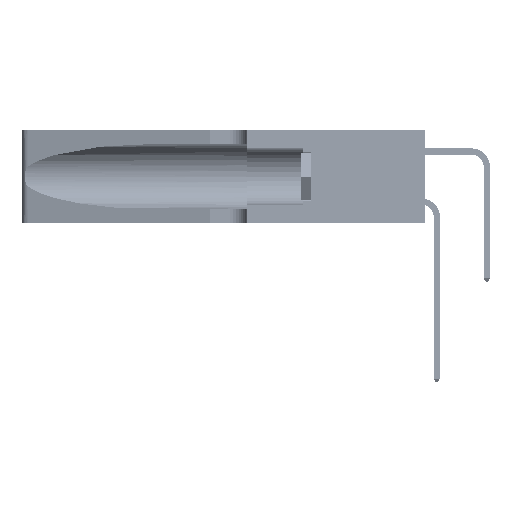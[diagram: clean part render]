
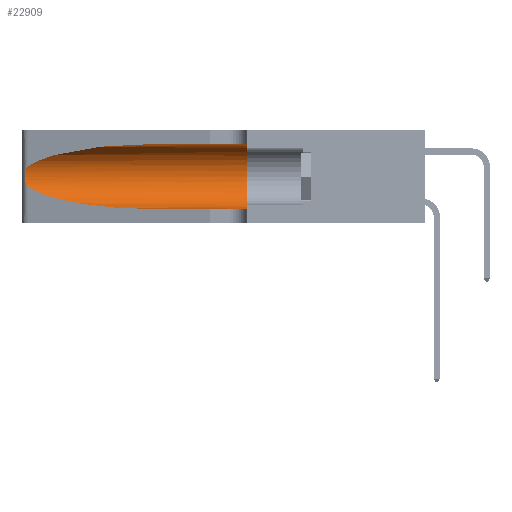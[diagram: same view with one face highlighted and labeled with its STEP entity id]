
A CAD part, left-side view. The second image highlights one B-rep face of the part: STEP entity #22909.
In plain terms, the highlighted cylindrical face has radius 3.308 mm (diameter 6.617 mm), a partial arc.
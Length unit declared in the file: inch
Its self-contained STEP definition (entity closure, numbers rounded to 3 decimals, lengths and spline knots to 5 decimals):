
#2068 = CARTESIAN_POINT ( 'NONE',  ( 0.1305, 0.72297, 0.31525 ) ) ;
#3001 = EDGE_CURVE ( 'NONE', #6214, #47529, #3493, .T. ) ;
#3493 = LINE ( 'NONE', #22109, #23967 ) ;
#3880 = EDGE_LOOP ( 'NONE', ( #43766, #30658, #31032, #28492, #28447, #49225 ) ) ;
#4367 = DIRECTION ( 'NONE',  ( 0., 1., 0. ) ) ;
#6214 = VERTEX_POINT ( 'NONE', #25042 ) ;
#7137 = CARTESIAN_POINT ( 'NONE',  ( 0.25787, 1.23484, 0.2124 ) ) ;
#8154 = AXIS2_PLACEMENT_3D ( 'NONE', #9022, #31868, #46830 ) ;
#8337 = CARTESIAN_POINT ( 'NONE',  ( 0.2373, 1.15595, 0.08982 ) ) ;
#9022 = CARTESIAN_POINT ( 'NONE',  ( 0.1305, 1.61858, 0.185 ) ) ;
#9195 = EDGE_CURVE ( 'NONE', #19633, #44971, #27323, .T. ) ;
#10660 = CIRCLE ( 'NONE', #34791, 0.13025 ) ;
#10864 = CARTESIAN_POINT ( 'NONE',  ( 0.25555, 1.22994, 0.2215 ) ) ;
#11026 = CARTESIAN_POINT ( 'NONE',  ( 0.26018, 1.23835, 0.19895 ) ) ;
#11902 = EDGE_CURVE ( 'NONE', #19633, #40848, #29176, .T. ) ;
#12067 = CARTESIAN_POINT ( 'NONE',  ( 0.1305, 0.72297, 0.31525 ) ) ;
#13399 = EDGE_CURVE ( 'NONE', #40848, #29617, #20331, .T. ) ;
#13569 = CARTESIAN_POINT ( 'NONE',  ( 0.2373, 1.15595, 0.28018 ) ) ;
#14860 = CARTESIAN_POINT ( 'NONE',  ( 0.26075, 1.23896, 0.178 ) ) ;
#16056 = CARTESIAN_POINT ( 'NONE',  ( 0.18966, 0.96281, 0.05475 ) ) ;
#18732 = CARTESIAN_POINT ( 'NONE',  ( 0.25856, 1.23593, 0.16098 ) ) ;
#19633 = VERTEX_POINT ( 'NONE', #12067 ) ;
#20220 = FACE_OUTER_BOUND ( 'NONE', #3880, .T. ) ;
#20252 = CARTESIAN_POINT ( 'NONE',  ( 0.1305, 0.35, 0.31525 ) ) ;
#20331 = B_SPLINE_CURVE_WITH_KNOTS ( 'NONE', 3,
 ( #22387, #10864, #30011, #7137, #33815, #11026, #37643, #14860, #41413, #18732, #45163, #22551, #48908, #26391 ),
 .UNSPECIFIED., .F., .F.,
 ( 4, 2, 2, 2, 2, 2, 4 ),
 ( 0., 0.00027, 0.00053, 0.00107, 0.0016, 0.00187, 0.00214 ),
 .UNSPECIFIED. ) ;
#20970 = CARTESIAN_POINT ( 'NONE',  ( 0.1305, 1.61858, 0.31525 ) ) ;
#22109 = CARTESIAN_POINT ( 'NONE',  ( 0.1305, 1.61858, 0.05475 ) ) ;
#22387 = CARTESIAN_POINT ( 'NONE',  ( 0.25487, 1.22718, 0.22369 ) ) ;
#22551 = CARTESIAN_POINT ( 'NONE',  ( 0.25639, 1.23186, 0.15144 ) ) ;
#22909 = ADVANCED_FACE ( 'NONE', ( #20220 ), #29135, .F. ) ;
#23967 = VECTOR ( 'NONE', #48482, 39.37008 ) ;
#25042 = CARTESIAN_POINT ( 'NONE',  ( 0.1305, 0.72297, 0.05475 ) ) ;
#26391 = CARTESIAN_POINT ( 'NONE',  ( 0.25487, 1.22718, 0.14631 ) ) ;
#27323 = LINE ( 'NONE', #20970, #46173 ) ;
#27332 = CARTESIAN_POINT ( 'NONE',  ( 0.1305, 0.35, 0.185 ) ) ;
#28430 = EDGE_CURVE ( 'NONE', #44971, #47529, #10660, .T. ) ;
#28447 = ORIENTED_EDGE ( 'NONE', *, *, #28430, .F. ) ;
#28492 = ORIENTED_EDGE ( 'NONE', *, *, #3001, .T. ) ;
#28885 = CARTESIAN_POINT ( 'NONE',  ( 0.25487, 1.22718, 0.22369 ) ) ;
#29135 = CYLINDRICAL_SURFACE ( 'NONE', #8154, 0.13025 ) ;
#29176 =( BOUNDED_CURVE ( )  B_SPLINE_CURVE ( 3, ( #2068, #47637, #13569, #28885 ),
 .UNSPECIFIED., .F., .F. ) 
 B_SPLINE_CURVE_WITH_KNOTS ( ( 4, 4 ),
 ( 1.5708, 2.84003 ),
 .UNSPECIFIED. ) 
 CURVE ( )  GEOMETRIC_REPRESENTATION_ITEM ( )  RATIONAL_B_SPLINE_CURVE ( ( 1., 0.87, 0.87, 1. ) ) 
 REPRESENTATION_ITEM ( '' )  );
#29617 = VERTEX_POINT ( 'NONE', #45178 ) ;
#30011 = CARTESIAN_POINT ( 'NONE',  ( 0.25639, 1.23184, 0.21858 ) ) ;
#30658 = ORIENTED_EDGE ( 'NONE', *, *, #13399, .T. ) ;
#31032 = ORIENTED_EDGE ( 'NONE', *, *, #44923, .T. ) ;
#31121 = DIRECTION ( 'NONE',  ( 0., 0., 1. ) ) ;
#31868 = DIRECTION ( 'NONE',  ( 0., -1., 0. ) ) ;
#33815 = CARTESIAN_POINT ( 'NONE',  ( 0.25854, 1.2359, 0.20912 ) ) ;
#34791 = AXIS2_PLACEMENT_3D ( 'NONE', #27332, #4367, #31121 ) ;
#35000 = CARTESIAN_POINT ( 'NONE',  ( 0.25487, 1.22718, 0.14631 ) ) ;
#35840 =( BOUNDED_CURVE ( )  B_SPLINE_CURVE ( 3, ( #35000, #8337, #16056, #42578 ),
 .UNSPECIFIED., .F., .T. ) 
 B_SPLINE_CURVE_WITH_KNOTS ( ( 4, 4 ),
 ( 3.44316, 4.71239 ),
 .UNSPECIFIED. ) 
 CURVE ( )  GEOMETRIC_REPRESENTATION_ITEM ( )  RATIONAL_B_SPLINE_CURVE ( ( 1., 0.87, 0.87, 1. ) ) 
 REPRESENTATION_ITEM ( '' )  );
#37643 = CARTESIAN_POINT ( 'NONE',  ( 0.26075, 1.23896, 0.19203 ) ) ;
#40017 = CARTESIAN_POINT ( 'NONE',  ( 0.25487, 1.22718, 0.22369 ) ) ;
#40027 = DIRECTION ( 'NONE',  ( 0., -1., 0. ) ) ;
#40848 = VERTEX_POINT ( 'NONE', #40017 ) ;
#41413 = CARTESIAN_POINT ( 'NONE',  ( 0.26017, 1.23833, 0.17102 ) ) ;
#42578 = CARTESIAN_POINT ( 'NONE',  ( 0.1305, 0.72297, 0.05475 ) ) ;
#43397 = CARTESIAN_POINT ( 'NONE',  ( 0.1305, 0.35, 0.05475 ) ) ;
#43766 = ORIENTED_EDGE ( 'NONE', *, *, #11902, .T. ) ;
#44923 = EDGE_CURVE ( 'NONE', #29617, #6214, #35840, .T. ) ;
#44971 = VERTEX_POINT ( 'NONE', #20252 ) ;
#45163 = CARTESIAN_POINT ( 'NONE',  ( 0.25789, 1.23486, 0.15765 ) ) ;
#45178 = CARTESIAN_POINT ( 'NONE',  ( 0.25487, 1.22718, 0.14631 ) ) ;
#46173 = VECTOR ( 'NONE', #40027, 39.37008 ) ;
#46830 = DIRECTION ( 'NONE',  ( 0., 0., -1. ) ) ;
#47529 = VERTEX_POINT ( 'NONE', #43397 ) ;
#47637 = CARTESIAN_POINT ( 'NONE',  ( 0.18966, 0.96281, 0.31525 ) ) ;
#48482 = DIRECTION ( 'NONE',  ( 0., -1., 0. ) ) ;
#48908 = CARTESIAN_POINT ( 'NONE',  ( 0.25555, 1.22993, 0.14849 ) ) ;
#49225 = ORIENTED_EDGE ( 'NONE', *, *, #9195, .F. ) ;
